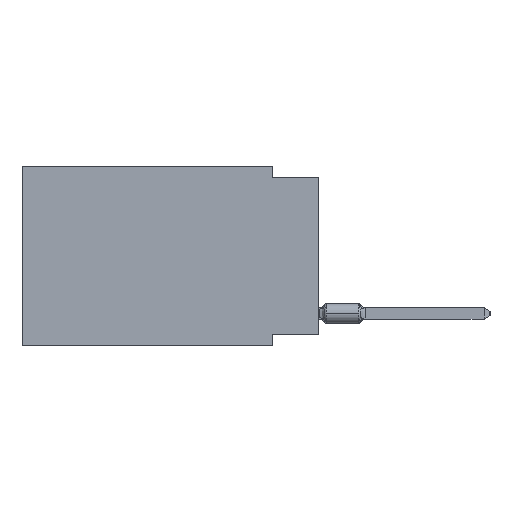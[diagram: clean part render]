
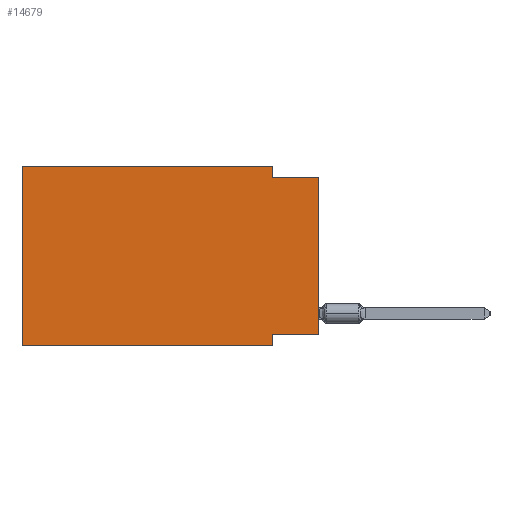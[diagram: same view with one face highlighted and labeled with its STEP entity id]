
A CAD part, left-side view. The second image highlights one B-rep face of the part: STEP entity #14679.
In plain terms, the highlighted planar face has unit normal (-1, 0, 0).
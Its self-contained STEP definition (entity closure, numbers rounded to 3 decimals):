
#368 = AXIS2_PLACEMENT_3D ( 'NONE', #11391, #76921, #30055 ) ;
#3125 = VECTOR ( 'NONE', #23130, 1000. ) ;
#3222 = DIRECTION ( 'NONE',  ( 0., 0., -1. ) ) ;
#5079 = CARTESIAN_POINT ( 'NONE',  ( 0., 0., -9.271 ) ) ;
#5752 = CARTESIAN_POINT ( 'NONE',  ( 0., 16.383, 0. ) ) ;
#6758 = LINE ( 'NONE', #36755, #24685 ) ;
#7078 = DIRECTION ( 'NONE',  ( 0., 0., 1. ) ) ;
#7107 = ORIENTED_EDGE ( 'NONE', *, *, #31280, .F. ) ;
#8961 = VERTEX_POINT ( 'NONE', #5752 ) ;
#10924 = ORIENTED_EDGE ( 'NONE', *, *, #50129, .T. ) ;
#11391 = CARTESIAN_POINT ( 'NONE',  ( 0., 16.383, 0. ) ) ;
#12601 = VERTEX_POINT ( 'NONE', #5079 ) ;
#13976 = ORIENTED_EDGE ( 'NONE', *, *, #15722, .F. ) ;
#13983 = VERTEX_POINT ( 'NONE', #54508 ) ;
#14003 = VECTOR ( 'NONE', #44267, 1000. ) ;
#14411 = CARTESIAN_POINT ( 'NONE',  ( 0., 2.54, -0.635 ) ) ;
#14679 = ADVANCED_FACE ( 'NONE', ( #29666 ), #64839, .F. ) ;
#15492 = CARTESIAN_POINT ( 'NONE',  ( 0., 2.54, -9.271 ) ) ;
#15696 = CARTESIAN_POINT ( 'NONE',  ( 0., 2.54, 0. ) ) ;
#15722 = EDGE_CURVE ( 'NONE', #66171, #29519, #21628, .T. ) ;
#16096 = VERTEX_POINT ( 'NONE', #39118 ) ;
#16601 = EDGE_LOOP ( 'NONE', ( #10924, #57531, #74992, #7107, #71213, #72160, #13976, #40817 ) ) ;
#16761 = DIRECTION ( 'NONE',  ( 0., -1., 0. ) ) ;
#18061 = DIRECTION ( 'NONE',  ( 0., -1., 0. ) ) ;
#19779 = VERTEX_POINT ( 'NONE', #47625 ) ;
#20649 = VECTOR ( 'NONE', #16761, 1000. ) ;
#21628 = LINE ( 'NONE', #32170, #14003 ) ;
#23130 = DIRECTION ( 'NONE',  ( 0., -1., 0. ) ) ;
#23331 = VERTEX_POINT ( 'NONE', #14411 ) ;
#24685 = VECTOR ( 'NONE', #18061, 1000. ) ;
#25809 = LINE ( 'NONE', #36377, #26120 ) ;
#26120 = VECTOR ( 'NONE', #72684, 1000. ) ;
#27144 = CARTESIAN_POINT ( 'NONE',  ( 0., 0., -0.635 ) ) ;
#29519 = VERTEX_POINT ( 'NONE', #42702 ) ;
#29666 = FACE_OUTER_BOUND ( 'NONE', #16601, .T. ) ;
#30055 = DIRECTION ( 'NONE',  ( 0., 0., -1. ) ) ;
#31280 = EDGE_CURVE ( 'NONE', #8961, #16096, #6758, .T. ) ;
#32170 = CARTESIAN_POINT ( 'NONE',  ( 0., 2.54, -9.906 ) ) ;
#36377 = CARTESIAN_POINT ( 'NONE',  ( 0., 0., 0. ) ) ;
#36755 = CARTESIAN_POINT ( 'NONE',  ( 0., 16.383, 0. ) ) ;
#39118 = CARTESIAN_POINT ( 'NONE',  ( 0., 2.54, 0. ) ) ;
#39209 = CARTESIAN_POINT ( 'NONE',  ( 0., 0., -9.271 ) ) ;
#40715 = VECTOR ( 'NONE', #7078, 1000. ) ;
#40817 = ORIENTED_EDGE ( 'NONE', *, *, #44801, .F. ) ;
#42702 = CARTESIAN_POINT ( 'NONE',  ( 0., 2.54, -9.906 ) ) ;
#44267 = DIRECTION ( 'NONE',  ( 0., 0., -1. ) ) ;
#44801 = EDGE_CURVE ( 'NONE', #12601, #66171, #57913, .T. ) ;
#45614 = LINE ( 'NONE', #45998, #20649 ) ;
#45998 = CARTESIAN_POINT ( 'NONE',  ( 0., 16.383, -9.906 ) ) ;
#46558 = LINE ( 'NONE', #27144, #3125 ) ;
#47625 = CARTESIAN_POINT ( 'NONE',  ( 0., 16.383, -9.906 ) ) ;
#49426 = VECTOR ( 'NONE', #3222, 1000. ) ;
#50129 = EDGE_CURVE ( 'NONE', #12601, #13983, #25809, .T. ) ;
#51296 = DIRECTION ( 'NONE',  ( 0., 1., 0. ) ) ;
#54270 = CARTESIAN_POINT ( 'NONE',  ( 0., 16.383, 0. ) ) ;
#54508 = CARTESIAN_POINT ( 'NONE',  ( 0., 0., -0.635 ) ) ;
#57531 = ORIENTED_EDGE ( 'NONE', *, *, #68850, .F. ) ;
#57913 = LINE ( 'NONE', #39209, #64602 ) ;
#64602 = VECTOR ( 'NONE', #51296, 1000. ) ;
#64839 = PLANE ( 'NONE',  #368 ) ;
#66171 = VERTEX_POINT ( 'NONE', #15492 ) ;
#68850 = EDGE_CURVE ( 'NONE', #23331, #13983, #46558, .T. ) ;
#69158 = LINE ( 'NONE', #15696, #49426 ) ;
#69449 = EDGE_CURVE ( 'NONE', #19779, #8961, #72635, .T. ) ;
#71213 = ORIENTED_EDGE ( 'NONE', *, *, #69449, .F. ) ;
#72160 = ORIENTED_EDGE ( 'NONE', *, *, #75278, .T. ) ;
#72635 = LINE ( 'NONE', #54270, #40715 ) ;
#72684 = DIRECTION ( 'NONE',  ( 0., 0., 1. ) ) ;
#74806 = EDGE_CURVE ( 'NONE', #16096, #23331, #69158, .T. ) ;
#74992 = ORIENTED_EDGE ( 'NONE', *, *, #74806, .F. ) ;
#75278 = EDGE_CURVE ( 'NONE', #19779, #29519, #45614, .T. ) ;
#76921 = DIRECTION ( 'NONE',  ( 1., 0., 0. ) ) ;
